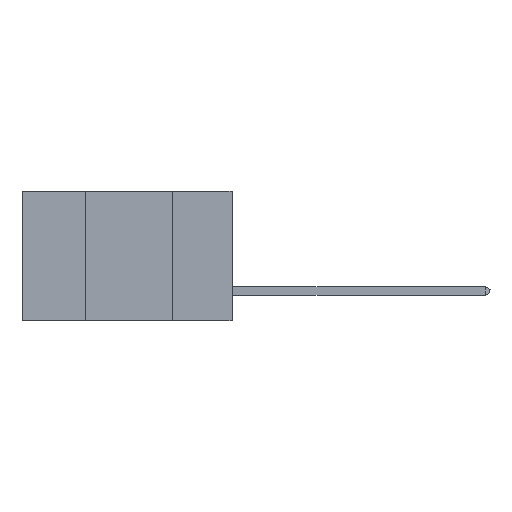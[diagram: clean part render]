
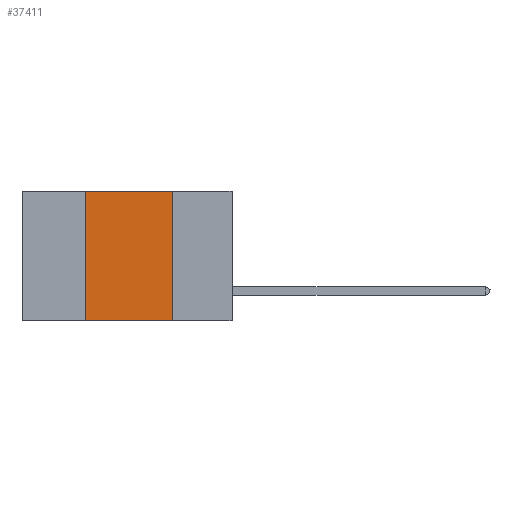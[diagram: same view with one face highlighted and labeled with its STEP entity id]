
A CAD part, left-side view. The second image highlights one B-rep face of the part: STEP entity #37411.
In plain terms, the highlighted planar face has unit normal (-1, 0, 0).
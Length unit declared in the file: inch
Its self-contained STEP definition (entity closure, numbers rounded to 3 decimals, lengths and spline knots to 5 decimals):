
#2942 = ORIENTED_EDGE ( 'NONE', *, *, #4288, .T. ) ;
#3064 = EDGE_LOOP ( 'NONE', ( #7829, #44648, #30337, #2942 ) ) ;
#4274 = VECTOR ( 'NONE', #41783, 39.37008 ) ;
#4288 = EDGE_CURVE ( 'NONE', #40728, #32188, #6521, .T. ) ;
#5267 = AXIS2_PLACEMENT_3D ( 'NONE', #39540, #32727, #12814 ) ;
#6521 = LINE ( 'NONE', #35276, #4274 ) ;
#7555 = FACE_OUTER_BOUND ( 'NONE', #3064, .T. ) ;
#7829 = ORIENTED_EDGE ( 'NONE', *, *, #15109, .F. ) ;
#12496 = CARTESIAN_POINT ( 'NONE',  ( 0., 0.17, 0. ) ) ;
#12814 = DIRECTION ( 'NONE',  ( 0., 0., -1. ) ) ;
#14478 = VERTEX_POINT ( 'NONE', #33280 ) ;
#15109 = EDGE_CURVE ( 'NONE', #34432, #32188, #39381, .T. ) ;
#15244 = PLANE ( 'NONE',  #5267 ) ;
#18307 = LINE ( 'NONE', #30137, #34035 ) ;
#18932 = DIRECTION ( 'NONE',  ( 0., -1., 0. ) ) ;
#20765 = LINE ( 'NONE', #42322, #23962 ) ;
#21656 = DIRECTION ( 'NONE',  ( 0., 0., 1. ) ) ;
#23962 = VECTOR ( 'NONE', #21656, 39.37008 ) ;
#29727 = VECTOR ( 'NONE', #41532, 39.37008 ) ;
#30137 = CARTESIAN_POINT ( 'NONE',  ( 0., 0.6, 0. ) ) ;
#30337 = ORIENTED_EDGE ( 'NONE', *, *, #36642, .F. ) ;
#32043 = CARTESIAN_POINT ( 'NONE',  ( 0., 0.17, -0.37 ) ) ;
#32188 = VERTEX_POINT ( 'NONE', #32043 ) ;
#32727 = DIRECTION ( 'NONE',  ( 1., 0., 0. ) ) ;
#33280 = CARTESIAN_POINT ( 'NONE',  ( 0., 0.42, 0. ) ) ;
#34035 = VECTOR ( 'NONE', #18932, 39.37008 ) ;
#34432 = VERTEX_POINT ( 'NONE', #12496 ) ;
#34610 = CARTESIAN_POINT ( 'NONE',  ( 0., 0.17, 0. ) ) ;
#35276 = CARTESIAN_POINT ( 'NONE',  ( 0., 0.6, -0.37 ) ) ;
#36642 = EDGE_CURVE ( 'NONE', #40728, #14478, #20765, .T. ) ;
#37411 = ADVANCED_FACE ( 'NONE', ( #7555 ), #15244, .F. ) ;
#38168 = EDGE_CURVE ( 'NONE', #14478, #34432, #18307, .T. ) ;
#39381 = LINE ( 'NONE', #34610, #29727 ) ;
#39540 = CARTESIAN_POINT ( 'NONE',  ( 0., 0.6, 0. ) ) ;
#40728 = VERTEX_POINT ( 'NONE', #43127 ) ;
#41532 = DIRECTION ( 'NONE',  ( 0., 0., -1. ) ) ;
#41783 = DIRECTION ( 'NONE',  ( 0., -1., 0. ) ) ;
#42322 = CARTESIAN_POINT ( 'NONE',  ( 0., 0.42, 0. ) ) ;
#43127 = CARTESIAN_POINT ( 'NONE',  ( 0., 0.42, -0.37 ) ) ;
#44648 = ORIENTED_EDGE ( 'NONE', *, *, #38168, .F. ) ;
